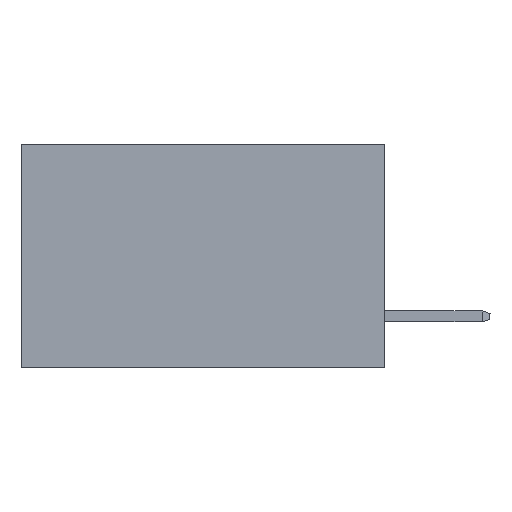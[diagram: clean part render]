
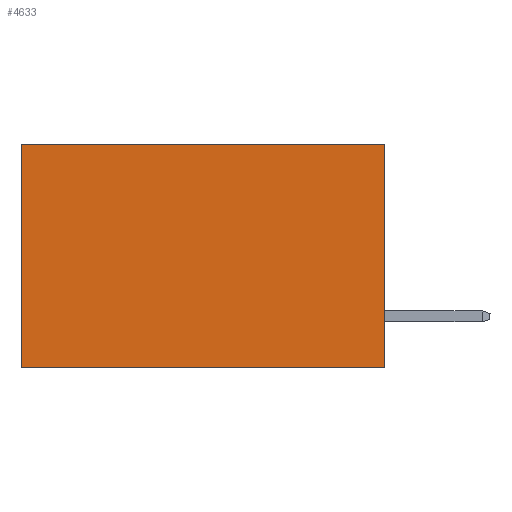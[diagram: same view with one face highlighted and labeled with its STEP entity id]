
A CAD part, left-side view. The second image highlights one B-rep face of the part: STEP entity #4633.
In plain terms, the highlighted planar face has unit normal (-1, 0, 0).
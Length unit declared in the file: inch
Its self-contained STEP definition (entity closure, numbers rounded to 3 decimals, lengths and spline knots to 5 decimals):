
#119 = AXIS2_PLACEMENT_3D ( 'NONE', #5917, #2869, #8228 ) ;
#603 = CARTESIAN_POINT ( 'NONE',  ( 0.2615, 0., -0.37 ) ) ;
#1074 = CARTESIAN_POINT ( 'NONE',  ( 0.2615, 0., 0. ) ) ;
#1120 = DIRECTION ( 'NONE',  ( 0., 1., 0. ) ) ;
#1304 = PLANE ( 'NONE',  #119 ) ;
#1324 = VECTOR ( 'NONE', #9091, 39.37008 ) ;
#1872 = LINE ( 'NONE', #2789, #8911 ) ;
#2765 = ORIENTED_EDGE ( 'NONE', *, *, #3610, .F. ) ;
#2775 = ORIENTED_EDGE ( 'NONE', *, *, #8503, .T. ) ;
#2789 = CARTESIAN_POINT ( 'NONE',  ( 0.2615, 0., -0.37 ) ) ;
#2869 = DIRECTION ( 'NONE',  ( 1., 0., 0. ) ) ;
#3073 = VECTOR ( 'NONE', #9695, 39.37008 ) ;
#3173 = CARTESIAN_POINT ( 'NONE',  ( 0.2615, 0., -0.37 ) ) ;
#3410 = EDGE_CURVE ( 'NONE', #7430, #5579, #6578, .T. ) ;
#3575 = CARTESIAN_POINT ( 'NONE',  ( 0.2615, 0.6, -0.37 ) ) ;
#3610 = EDGE_CURVE ( 'NONE', #5369, #7605, #6418, .T. ) ;
#3618 = LINE ( 'NONE', #4996, #1324 ) ;
#3749 = ORIENTED_EDGE ( 'NONE', *, *, #9374, .F. ) ;
#3981 = DIRECTION ( 'NONE',  ( 0., 0., -1. ) ) ;
#4633 = ADVANCED_FACE ( 'NONE', ( #6021 ), #1304, .F. ) ;
#4996 = CARTESIAN_POINT ( 'NONE',  ( 0.2615, 0., 0. ) ) ;
#5082 = EDGE_LOOP ( 'NONE', ( #5789, #3749, #2765, #2775 ) ) ;
#5369 = VERTEX_POINT ( 'NONE', #1074 ) ;
#5579 = VERTEX_POINT ( 'NONE', #7632 ) ;
#5789 = ORIENTED_EDGE ( 'NONE', *, *, #3410, .T. ) ;
#5917 = CARTESIAN_POINT ( 'NONE',  ( 0.2615, 0., -0.37 ) ) ;
#6021 = FACE_OUTER_BOUND ( 'NONE', #5082, .T. ) ;
#6418 = LINE ( 'NONE', #3173, #9589 ) ;
#6578 = LINE ( 'NONE', #3575, #3073 ) ;
#7430 = VERTEX_POINT ( 'NONE', #9133 ) ;
#7605 = VERTEX_POINT ( 'NONE', #603 ) ;
#7632 = CARTESIAN_POINT ( 'NONE',  ( 0.2615, 0.6, -0.37 ) ) ;
#8228 = DIRECTION ( 'NONE',  ( 0., 0., -1. ) ) ;
#8503 = EDGE_CURVE ( 'NONE', #5369, #7430, #3618, .T. ) ;
#8911 = VECTOR ( 'NONE', #1120, 39.37008 ) ;
#9091 = DIRECTION ( 'NONE',  ( 0., 1., 0. ) ) ;
#9133 = CARTESIAN_POINT ( 'NONE',  ( 0.2615, 0.6, 0. ) ) ;
#9374 = EDGE_CURVE ( 'NONE', #7605, #5579, #1872, .T. ) ;
#9589 = VECTOR ( 'NONE', #3981, 39.37008 ) ;
#9695 = DIRECTION ( 'NONE',  ( 0., 0., -1. ) ) ;
